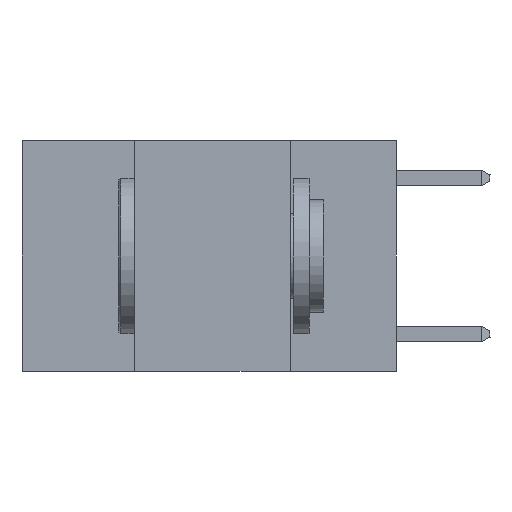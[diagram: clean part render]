
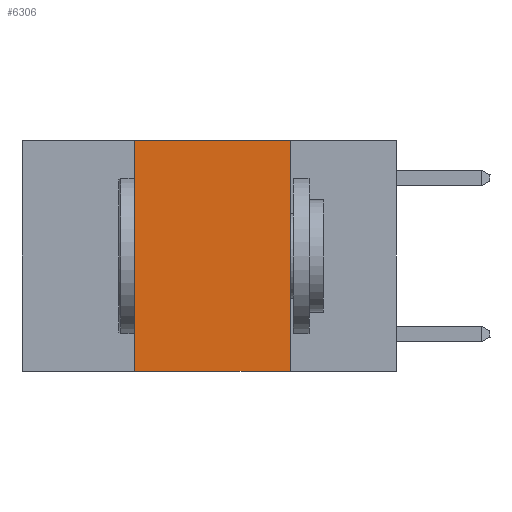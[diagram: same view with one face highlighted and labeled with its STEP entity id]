
A CAD part, left-side view. The second image highlights one B-rep face of the part: STEP entity #6306.
In plain terms, the highlighted planar face has unit normal (-1, 0, 0).
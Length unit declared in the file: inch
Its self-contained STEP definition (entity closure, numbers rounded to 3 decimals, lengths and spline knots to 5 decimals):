
#222 = ORIENTED_EDGE ( 'NONE', *, *, #4953, .F. ) ;
#877 = EDGE_CURVE ( 'NONE', #11410, #1471, #9988, .T. ) ;
#1471 = VERTEX_POINT ( 'NONE', #2300 ) ;
#2300 = CARTESIAN_POINT ( 'NONE',  ( 0., 0.17, -0.37 ) ) ;
#2302 = VECTOR ( 'NONE', #6518, 39.37008 ) ;
#3100 = CARTESIAN_POINT ( 'NONE',  ( 0., 0.6, -0.37 ) ) ;
#3583 = DIRECTION ( 'NONE',  ( 0., 0., -1. ) ) ;
#4166 = VERTEX_POINT ( 'NONE', #19671 ) ;
#4953 = EDGE_CURVE ( 'NONE', #11410, #4166, #18636, .T. ) ;
#5085 = DIRECTION ( 'NONE',  ( 1., 0., 0. ) ) ;
#5199 = ORIENTED_EDGE ( 'NONE', *, *, #5305, .F. ) ;
#5305 = EDGE_CURVE ( 'NONE', #10467, #1471, #8825, .T. ) ;
#5659 = LINE ( 'NONE', #9326, #11666 ) ;
#6306 = ADVANCED_FACE ( 'NONE', ( #18552 ), #20309, .F. ) ;
#6518 = DIRECTION ( 'NONE',  ( 0., -1., 0. ) ) ;
#8436 = CARTESIAN_POINT ( 'NONE',  ( 0., 0.6, 0. ) ) ;
#8528 = CARTESIAN_POINT ( 'NONE',  ( 0., 0.42, 0. ) ) ;
#8825 = LINE ( 'NONE', #13520, #12023 ) ;
#9326 = CARTESIAN_POINT ( 'NONE',  ( 0., 0.6, 0. ) ) ;
#9988 = LINE ( 'NONE', #3100, #2302 ) ;
#10039 = EDGE_CURVE ( 'NONE', #4166, #10467, #5659, .T. ) ;
#10467 = VERTEX_POINT ( 'NONE', #20834 ) ;
#11410 = VERTEX_POINT ( 'NONE', #17136 ) ;
#11661 = EDGE_LOOP ( 'NONE', ( #5199, #20392, #222, #12470 ) ) ;
#11666 = VECTOR ( 'NONE', #20969, 39.37008 ) ;
#12023 = VECTOR ( 'NONE', #3583, 39.37008 ) ;
#12470 = ORIENTED_EDGE ( 'NONE', *, *, #877, .T. ) ;
#12553 = AXIS2_PLACEMENT_3D ( 'NONE', #8436, #5085, #17100 ) ;
#13520 = CARTESIAN_POINT ( 'NONE',  ( 0., 0.17, 0. ) ) ;
#13768 = DIRECTION ( 'NONE',  ( 0., 0., 1. ) ) ;
#17100 = DIRECTION ( 'NONE',  ( 0., 0., -1. ) ) ;
#17136 = CARTESIAN_POINT ( 'NONE',  ( 0., 0.42, -0.37 ) ) ;
#18552 = FACE_OUTER_BOUND ( 'NONE', #11661, .T. ) ;
#18636 = LINE ( 'NONE', #8528, #19703 ) ;
#19671 = CARTESIAN_POINT ( 'NONE',  ( 0., 0.42, 0. ) ) ;
#19703 = VECTOR ( 'NONE', #13768, 39.37008 ) ;
#20309 = PLANE ( 'NONE',  #12553 ) ;
#20392 = ORIENTED_EDGE ( 'NONE', *, *, #10039, .F. ) ;
#20834 = CARTESIAN_POINT ( 'NONE',  ( 0., 0.17, 0. ) ) ;
#20969 = DIRECTION ( 'NONE',  ( 0., -1., 0. ) ) ;
